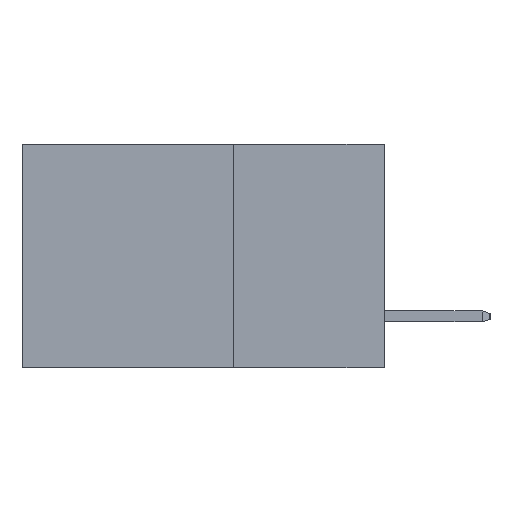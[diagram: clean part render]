
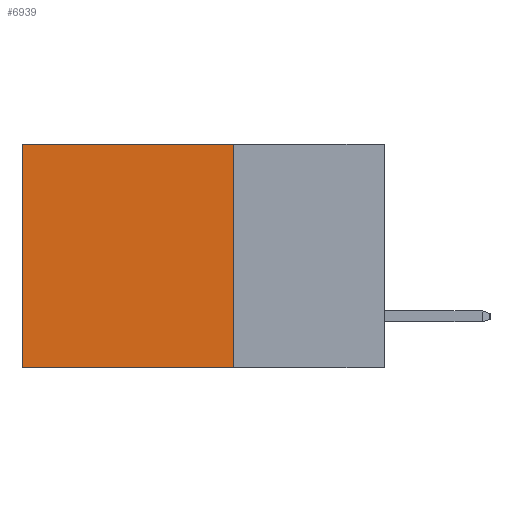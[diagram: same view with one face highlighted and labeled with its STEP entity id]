
A CAD part, left-side view. The second image highlights one B-rep face of the part: STEP entity #6939.
In plain terms, the highlighted planar face has unit normal (-1, 0, 0).
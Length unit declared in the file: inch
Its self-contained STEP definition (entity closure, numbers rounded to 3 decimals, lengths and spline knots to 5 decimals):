
#489 = CARTESIAN_POINT ( 'NONE',  ( 0.2615, 0.6, -0.37 ) ) ;
#619 = CARTESIAN_POINT ( 'NONE',  ( 0.2615, 0.25, -0.37 ) ) ;
#1902 = DIRECTION ( 'NONE',  ( 0., 0., -1. ) ) ;
#2619 = EDGE_CURVE ( 'NONE', #3294, #9806, #16671, .T. ) ;
#3294 = VERTEX_POINT ( 'NONE', #9561 ) ;
#3308 = CARTESIAN_POINT ( 'NONE',  ( 0.2615, 0.25, -0.37 ) ) ;
#3352 = EDGE_CURVE ( 'NONE', #6964, #3294, #7537, .T. ) ;
#3515 = DIRECTION ( 'NONE',  ( 0., 1., 0. ) ) ;
#3890 = VERTEX_POINT ( 'NONE', #5543 ) ;
#4053 = VECTOR ( 'NONE', #4639, 39.37008 ) ;
#4639 = DIRECTION ( 'NONE',  ( 0., 0., -1. ) ) ;
#4773 = DIRECTION ( 'NONE',  ( 0., 0., -1. ) ) ;
#4863 = ORIENTED_EDGE ( 'NONE', *, *, #16425, .T. ) ;
#5422 = CARTESIAN_POINT ( 'NONE',  ( 0.2615, 0.25, -0.37 ) ) ;
#5543 = CARTESIAN_POINT ( 'NONE',  ( 0.2615, 0.6, 0. ) ) ;
#6206 = DIRECTION ( 'NONE',  ( 0., 1., 0. ) ) ;
#6751 = VECTOR ( 'NONE', #6206, 39.37008 ) ;
#6764 = FACE_OUTER_BOUND ( 'NONE', #7300, .T. ) ;
#6939 = ADVANCED_FACE ( 'NONE', ( #6764 ), #16395, .F. ) ;
#6964 = VERTEX_POINT ( 'NONE', #15204 ) ;
#7300 = EDGE_LOOP ( 'NONE', ( #8484, #11315, #8909, #4863 ) ) ;
#7537 = LINE ( 'NONE', #5422, #4053 ) ;
#8380 = AXIS2_PLACEMENT_3D ( 'NONE', #619, #12619, #4773 ) ;
#8484 = ORIENTED_EDGE ( 'NONE', *, *, #14860, .T. ) ;
#8909 = ORIENTED_EDGE ( 'NONE', *, *, #3352, .F. ) ;
#9561 = CARTESIAN_POINT ( 'NONE',  ( 0.2615, 0.25, -0.37 ) ) ;
#9806 = VERTEX_POINT ( 'NONE', #16486 ) ;
#11315 = ORIENTED_EDGE ( 'NONE', *, *, #2619, .F. ) ;
#12619 = DIRECTION ( 'NONE',  ( 1., 0., 0. ) ) ;
#13324 = VECTOR ( 'NONE', #3515, 39.37008 ) ;
#13451 = VECTOR ( 'NONE', #1902, 39.37008 ) ;
#13978 = CARTESIAN_POINT ( 'NONE',  ( 0.2615, 0.25, 0. ) ) ;
#14115 = LINE ( 'NONE', #13978, #6751 ) ;
#14860 = EDGE_CURVE ( 'NONE', #3890, #9806, #16801, .T. ) ;
#15204 = CARTESIAN_POINT ( 'NONE',  ( 0.2615, 0.25, 0. ) ) ;
#16395 = PLANE ( 'NONE',  #8380 ) ;
#16425 = EDGE_CURVE ( 'NONE', #6964, #3890, #14115, .T. ) ;
#16486 = CARTESIAN_POINT ( 'NONE',  ( 0.2615, 0.6, -0.37 ) ) ;
#16671 = LINE ( 'NONE', #3308, #13324 ) ;
#16801 = LINE ( 'NONE', #489, #13451 ) ;
